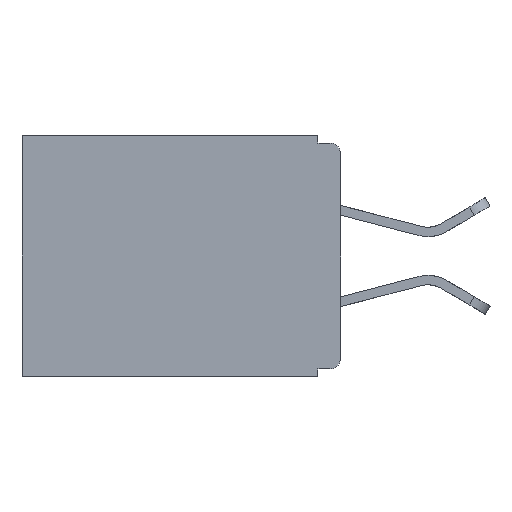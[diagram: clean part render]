
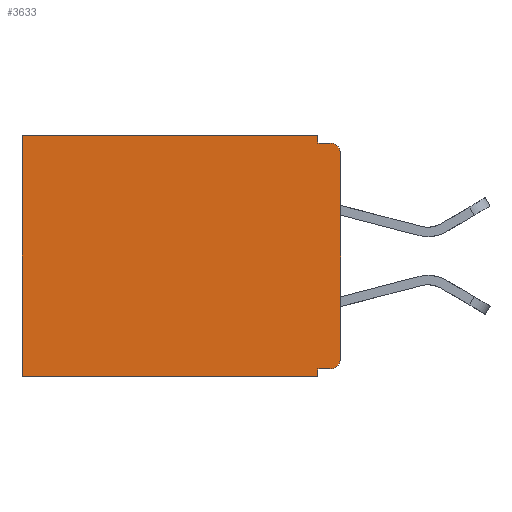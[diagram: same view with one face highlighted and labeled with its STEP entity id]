
A CAD part, left-side view. The second image highlights one B-rep face of the part: STEP entity #3633.
In plain terms, the highlighted planar face has unit normal (-1, 0, 0).
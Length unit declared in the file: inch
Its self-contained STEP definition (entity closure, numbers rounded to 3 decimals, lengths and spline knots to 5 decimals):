
#340 = VERTEX_POINT ( 'NONE', #15664 ) ;
#415 = VERTEX_POINT ( 'NONE', #12073 ) ;
#807 = ORIENTED_EDGE ( 'NONE', *, *, #11658, .F. ) ;
#909 = VERTEX_POINT ( 'NONE', #4775 ) ;
#980 = CARTESIAN_POINT ( 'NONE',  ( 0.3, 0.437, -0.33 ) ) ;
#1152 = DIRECTION ( 'NONE',  ( -1., 0., 0. ) ) ;
#1423 = CARTESIAN_POINT ( 'NONE',  ( 0.3, 0., -0.025 ) ) ;
#1562 = VERTEX_POINT ( 'NONE', #12438 ) ;
#1722 = VERTEX_POINT ( 'NONE', #1423 ) ;
#1944 = CIRCLE ( 'NONE', #13077, 0.015 ) ;
#2036 = DIRECTION ( 'NONE',  ( 0., 1., 0. ) ) ;
#2101 = DIRECTION ( 'NONE',  ( -1., 0., 0. ) ) ;
#2555 = ORIENTED_EDGE ( 'NONE', *, *, #5050, .F. ) ;
#3016 = EDGE_CURVE ( 'NONE', #1722, #4648, #1944, .T. ) ;
#3524 = EDGE_CURVE ( 'NONE', #10632, #4767, #5083, .T. ) ;
#3633 = ADVANCED_FACE ( 'NONE', ( #6464 ), #12878, .F. ) ;
#3865 = CARTESIAN_POINT ( 'NONE',  ( 0.3, 0.015, -0.025 ) ) ;
#4118 = ORIENTED_EDGE ( 'NONE', *, *, #6907, .T. ) ;
#4264 = ORIENTED_EDGE ( 'NONE', *, *, #12769, .T. ) ;
#4637 = ORIENTED_EDGE ( 'NONE', *, *, #15070, .T. ) ;
#4648 = VERTEX_POINT ( 'NONE', #9197 ) ;
#4670 = VECTOR ( 'NONE', #2036, 39.37008 ) ;
#4767 = VERTEX_POINT ( 'NONE', #9597 ) ;
#4775 = CARTESIAN_POINT ( 'NONE',  ( 0.3, 0., -0.305 ) ) ;
#4784 = CARTESIAN_POINT ( 'NONE',  ( 0.3, 0., -0.32 ) ) ;
#5050 = EDGE_CURVE ( 'NONE', #9893, #12451, #16570, .T. ) ;
#5083 = LINE ( 'NONE', #4784, #4670 ) ;
#5415 = LINE ( 'NONE', #7670, #15010 ) ;
#5808 = VECTOR ( 'NONE', #9774, 39.37008 ) ;
#6276 = LINE ( 'NONE', #14795, #15851 ) ;
#6464 = FACE_OUTER_BOUND ( 'NONE', #9094, .T. ) ;
#6798 = CARTESIAN_POINT ( 'NONE',  ( 0.3, 0.031, 0. ) ) ;
#6907 = EDGE_CURVE ( 'NONE', #9893, #340, #15367, .T. ) ;
#7192 = VECTOR ( 'NONE', #10091, 39.37008 ) ;
#7595 = DIRECTION ( 'NONE',  ( 0., -1., 0. ) ) ;
#7670 = CARTESIAN_POINT ( 'NONE',  ( 0.3, 0., -0.33 ) ) ;
#8680 = CARTESIAN_POINT ( 'NONE',  ( 0.3, 0., 0. ) ) ;
#9094 = EDGE_LOOP ( 'NONE', ( #13626, #9328, #13157, #2555, #4118, #4637, #807, #12427, #9248, #4264 ) ) ;
#9193 = LINE ( 'NONE', #14700, #5808 ) ;
#9197 = CARTESIAN_POINT ( 'NONE',  ( 0.3, 0.015, -0.01 ) ) ;
#9248 = ORIENTED_EDGE ( 'NONE', *, *, #3524, .F. ) ;
#9328 = ORIENTED_EDGE ( 'NONE', *, *, #3016, .T. ) ;
#9597 = CARTESIAN_POINT ( 'NONE',  ( 0.3, 0.031, -0.32 ) ) ;
#9774 = DIRECTION ( 'NONE',  ( 0., 0., -1. ) ) ;
#9873 = CARTESIAN_POINT ( 'NONE',  ( 0.3, 0.015, -0.305 ) ) ;
#9893 = VERTEX_POINT ( 'NONE', #6798 ) ;
#10091 = DIRECTION ( 'NONE',  ( 0., 0., -1. ) ) ;
#10177 = LINE ( 'NONE', #980, #7192 ) ;
#10632 = VERTEX_POINT ( 'NONE', #14328 ) ;
#10691 = LINE ( 'NONE', #15078, #13596 ) ;
#10822 = VECTOR ( 'NONE', #15812, 39.37008 ) ;
#11139 = DIRECTION ( 'NONE',  ( 0., 0., -1. ) ) ;
#11443 = DIRECTION ( 'NONE',  ( 0., 1., 0. ) ) ;
#11658 = EDGE_CURVE ( 'NONE', #415, #1562, #10691, .T. ) ;
#12073 = CARTESIAN_POINT ( 'NONE',  ( 0.3, 0.031, -0.33 ) ) ;
#12427 = ORIENTED_EDGE ( 'NONE', *, *, #14907, .F. ) ;
#12438 = CARTESIAN_POINT ( 'NONE',  ( 0.3, 0.437, -0.33 ) ) ;
#12451 = VERTEX_POINT ( 'NONE', #12903 ) ;
#12534 = VECTOR ( 'NONE', #14157, 39.37008 ) ;
#12769 = EDGE_CURVE ( 'NONE', #10632, #909, #13374, .T. ) ;
#12782 = EDGE_CURVE ( 'NONE', #12451, #4648, #6276, .T. ) ;
#12878 = PLANE ( 'NONE',  #14095 ) ;
#12903 = CARTESIAN_POINT ( 'NONE',  ( 0.3, 0.031, -0.01 ) ) ;
#13077 = AXIS2_PLACEMENT_3D ( 'NONE', #3865, #1152, #14474 ) ;
#13157 = ORIENTED_EDGE ( 'NONE', *, *, #12782, .F. ) ;
#13226 = AXIS2_PLACEMENT_3D ( 'NONE', #9873, #2101, #11139 ) ;
#13374 = CIRCLE ( 'NONE', #13226, 0.015 ) ;
#13571 = CARTESIAN_POINT ( 'NONE',  ( 0.3, 0.031, 0. ) ) ;
#13596 = VECTOR ( 'NONE', #11443, 39.37008 ) ;
#13626 = ORIENTED_EDGE ( 'NONE', *, *, #14518, .F. ) ;
#13918 = DIRECTION ( 'NONE',  ( 1., 0., 0. ) ) ;
#14095 = AXIS2_PLACEMENT_3D ( 'NONE', #14370, #13918, #14159 ) ;
#14157 = DIRECTION ( 'NONE',  ( 0., 1., 0. ) ) ;
#14159 = DIRECTION ( 'NONE',  ( 0., 0., -1. ) ) ;
#14328 = CARTESIAN_POINT ( 'NONE',  ( 0.3, 0.015, -0.32 ) ) ;
#14370 = CARTESIAN_POINT ( 'NONE',  ( 0.3, 0., -0.33 ) ) ;
#14474 = DIRECTION ( 'NONE',  ( 0., 0., -1. ) ) ;
#14518 = EDGE_CURVE ( 'NONE', #1722, #909, #5415, .T. ) ;
#14700 = CARTESIAN_POINT ( 'NONE',  ( 0.3, 0.031, -0.33 ) ) ;
#14795 = CARTESIAN_POINT ( 'NONE',  ( 0.3, 0., -0.01 ) ) ;
#14907 = EDGE_CURVE ( 'NONE', #4767, #415, #9193, .T. ) ;
#15010 = VECTOR ( 'NONE', #15123, 39.37008 ) ;
#15070 = EDGE_CURVE ( 'NONE', #340, #1562, #10177, .T. ) ;
#15078 = CARTESIAN_POINT ( 'NONE',  ( 0.3, 0., -0.33 ) ) ;
#15123 = DIRECTION ( 'NONE',  ( 0., 0., -1. ) ) ;
#15367 = LINE ( 'NONE', #8680, #12534 ) ;
#15664 = CARTESIAN_POINT ( 'NONE',  ( 0.3, 0.437, 0. ) ) ;
#15812 = DIRECTION ( 'NONE',  ( 0., 0., -1. ) ) ;
#15851 = VECTOR ( 'NONE', #7595, 39.37008 ) ;
#16570 = LINE ( 'NONE', #13571, #10822 ) ;
